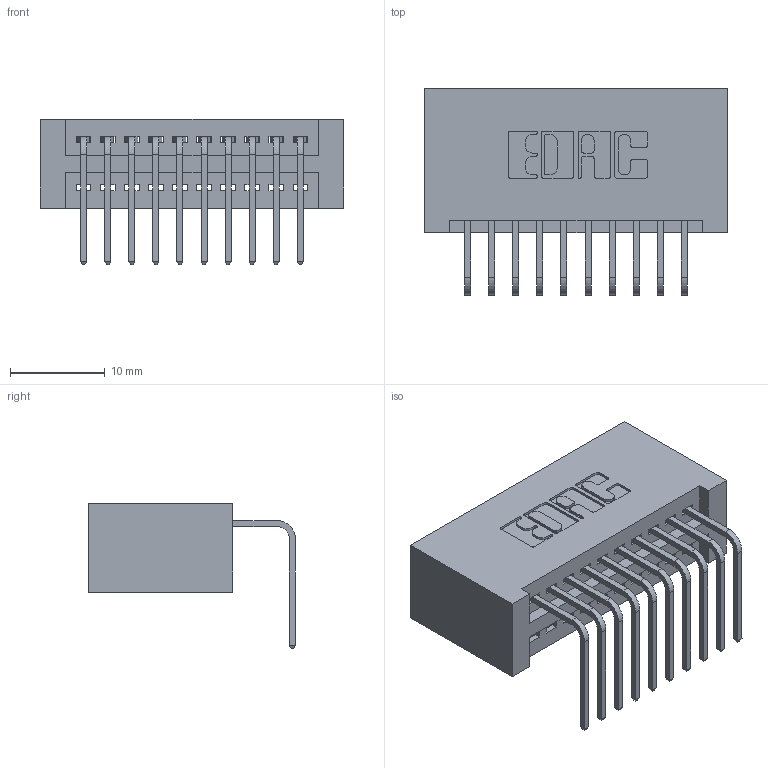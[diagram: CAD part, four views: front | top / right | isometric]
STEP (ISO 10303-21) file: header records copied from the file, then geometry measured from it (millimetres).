
FILE_DESCRIPTION (( 'STEP AP203' ), '1' );
FILE_NAME ('345-010-558-101.STEP', '2019-10-10T11:19:17', ( '' ), ( '' ), 'SwSTEP 2.0', 'SolidWorks 2016', '' );
FILE_SCHEMA (( 'CONFIG_CONTROL_DESIGN' ));
Length unit declared in the file: inch
Products named in the file (3): 345 Part_No Mounting Lugs; 345-292-001_558 Tail - 2; 345-010-558-101
Assembly tree (11 placements, depth 2):
  345-010-558-101
    345 Part_No Mounting Lugs
    345-292-001_558 Tail - 2  x10
Bounding box: 32 x 21.83 x 15.37 mm (x, y, z)
Volume: 3395.3 mm3; surface area: 4463.1 mm2
Topology: 11 solids, 11 shells, 718 faces, 2137 edges, 1410 vertices
Faces by surface type: plane 496, cylinder 222
Entity records: 11641 total; most frequent: CARTESIAN_POINT 2026, ORIENTED_EDGE 1970, DIRECTION 1809, EDGE_CURVE 985, LINE 821, VECTOR 821, VERTEX_POINT 654, AXIS2_PLACEMENT_3D 494
